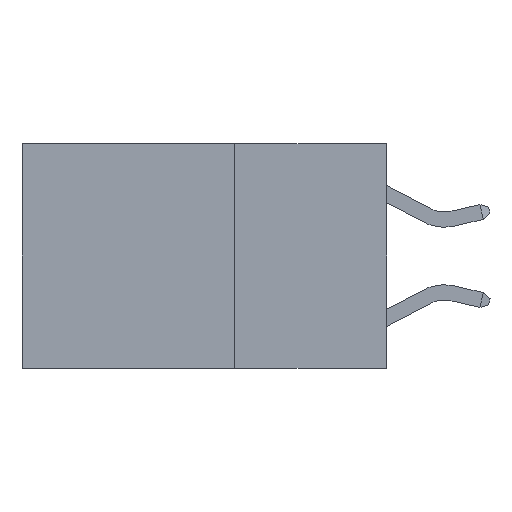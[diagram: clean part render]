
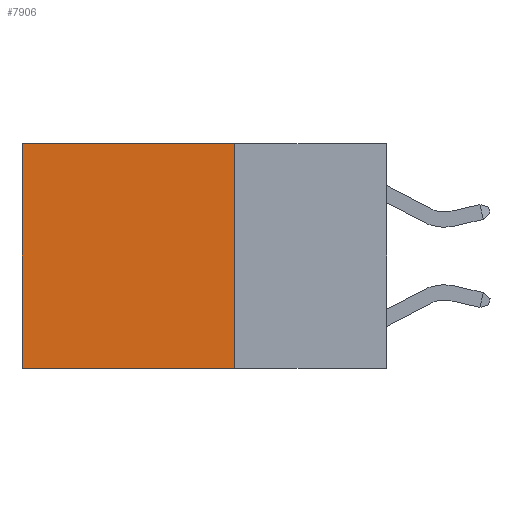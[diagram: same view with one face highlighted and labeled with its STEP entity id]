
A CAD part, left-side view. The second image highlights one B-rep face of the part: STEP entity #7906.
In plain terms, the highlighted planar face has unit normal (-1, 0, 0).
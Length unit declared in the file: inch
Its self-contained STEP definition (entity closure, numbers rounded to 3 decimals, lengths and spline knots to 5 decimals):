
#3 = CARTESIAN_POINT ( 'NONE',  ( 0.2625, 0.25, -0.37 ) ) ;
#207 = EDGE_CURVE ( 'NONE', #3862, #8748, #5128, .T. ) ;
#238 = CARTESIAN_POINT ( 'NONE',  ( 0.2625, 0.6, -0.37 ) ) ;
#337 = DIRECTION ( 'NONE',  ( 0., 0., -1. ) ) ;
#1053 = DIRECTION ( 'NONE',  ( 1., 0., 0. ) ) ;
#1293 = EDGE_CURVE ( 'NONE', #6813, #4051, #6465, .T. ) ;
#1693 = LINE ( 'NONE', #5196, #6853 ) ;
#2414 = CARTESIAN_POINT ( 'NONE',  ( 0.2625, 0.6, 0. ) ) ;
#2440 = CARTESIAN_POINT ( 'NONE',  ( 0.2625, 0.25, -0.37 ) ) ;
#3371 = FACE_OUTER_BOUND ( 'NONE', #3912, .T. ) ;
#3502 = LINE ( 'NONE', #2440, #5458 ) ;
#3550 = CARTESIAN_POINT ( 'NONE',  ( 0.2625, 0.25, 0. ) ) ;
#3701 = EDGE_CURVE ( 'NONE', #3862, #6813, #1693, .T. ) ;
#3707 = DIRECTION ( 'NONE',  ( 0., 0., -1. ) ) ;
#3813 = CARTESIAN_POINT ( 'NONE',  ( 0.2625, 0.25, 0. ) ) ;
#3862 = VERTEX_POINT ( 'NONE', #3550 ) ;
#3912 = EDGE_LOOP ( 'NONE', ( #7670, #7725, #7853, #7877 ) ) ;
#4051 = VERTEX_POINT ( 'NONE', #238 ) ;
#4173 = EDGE_CURVE ( 'NONE', #8748, #4051, #3502, .T. ) ;
#4677 = VECTOR ( 'NONE', #3707, 39.37008 ) ;
#5128 = LINE ( 'NONE', #3813, #6290 ) ;
#5172 = DIRECTION ( 'NONE',  ( 0., 0., -1. ) ) ;
#5196 = CARTESIAN_POINT ( 'NONE',  ( 0.2625, 0.25, 0. ) ) ;
#5231 = DIRECTION ( 'NONE',  ( 0., 1., 0. ) ) ;
#5458 = VECTOR ( 'NONE', #6379, 39.37008 ) ;
#6290 = VECTOR ( 'NONE', #5172, 39.37008 ) ;
#6379 = DIRECTION ( 'NONE',  ( 0., 1., 0. ) ) ;
#6465 = LINE ( 'NONE', #2414, #4677 ) ;
#6813 = VERTEX_POINT ( 'NONE', #8690 ) ;
#6853 = VECTOR ( 'NONE', #5231, 39.37008 ) ;
#7670 = ORIENTED_EDGE ( 'NONE', *, *, #1293, .T. ) ;
#7725 = ORIENTED_EDGE ( 'NONE', *, *, #4173, .F. ) ;
#7833 = CARTESIAN_POINT ( 'NONE',  ( 0.2625, 0.25, 0. ) ) ;
#7853 = ORIENTED_EDGE ( 'NONE', *, *, #207, .F. ) ;
#7877 = ORIENTED_EDGE ( 'NONE', *, *, #3701, .T. ) ;
#7906 = ADVANCED_FACE ( 'NONE', ( #3371 ), #8506, .F. ) ;
#8251 = AXIS2_PLACEMENT_3D ( 'NONE', #7833, #1053, #337 ) ;
#8506 = PLANE ( 'NONE',  #8251 ) ;
#8690 = CARTESIAN_POINT ( 'NONE',  ( 0.2625, 0.6, 0. ) ) ;
#8748 = VERTEX_POINT ( 'NONE', #3 ) ;
